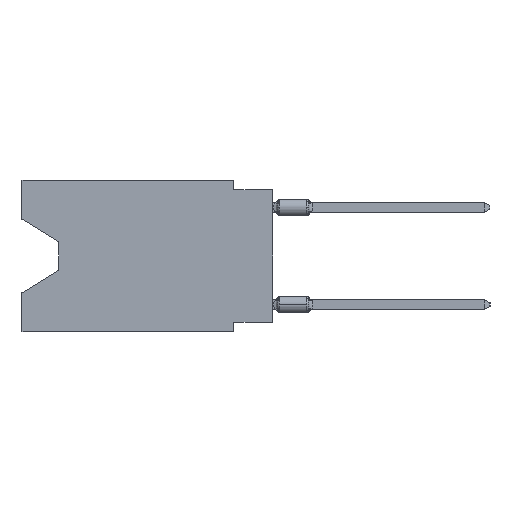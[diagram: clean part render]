
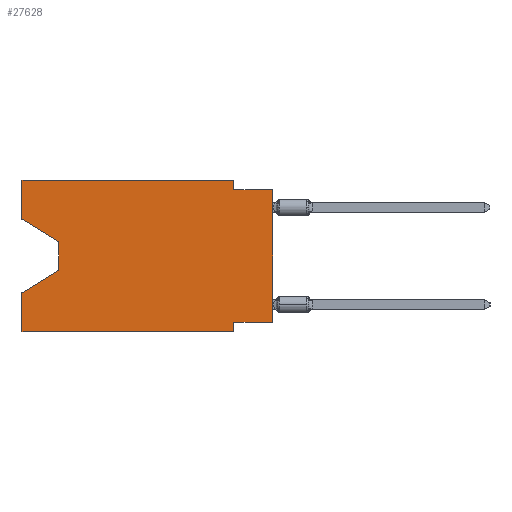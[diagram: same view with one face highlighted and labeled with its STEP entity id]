
A CAD part, left-side view. The second image highlights one B-rep face of the part: STEP entity #27628.
In plain terms, the highlighted planar face has unit normal (-1, 0, 0).
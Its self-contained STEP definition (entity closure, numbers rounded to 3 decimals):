
#30 = LINE ( 'NONE', #31520, #30660 ) ;
#579 = VECTOR ( 'NONE', #12243, 1000. ) ;
#632 = EDGE_CURVE ( 'NONE', #50674, #3811, #5623, .T. ) ;
#1959 = CARTESIAN_POINT ( 'NONE',  ( 0., 16.383, 0. ) ) ;
#2284 = VECTOR ( 'NONE', #51133, 1000. ) ;
#2565 = VERTEX_POINT ( 'NONE', #56845 ) ;
#3761 = EDGE_CURVE ( 'NONE', #54432, #61851, #59357, .T. ) ;
#3811 = VERTEX_POINT ( 'NONE', #17950 ) ;
#4368 = ORIENTED_EDGE ( 'NONE', *, *, #3761, .F. ) ;
#5499 = CARTESIAN_POINT ( 'NONE',  ( 0., 13.97, -4.013 ) ) ;
#5519 = VERTEX_POINT ( 'NONE', #28139 ) ;
#5593 = ORIENTED_EDGE ( 'NONE', *, *, #47356, .F. ) ;
#5623 = LINE ( 'NONE', #37095, #46835 ) ;
#8354 = CARTESIAN_POINT ( 'NONE',  ( 0., 0., -9.271 ) ) ;
#8778 = EDGE_CURVE ( 'NONE', #24828, #60462, #59482, .T. ) ;
#9676 = VECTOR ( 'NONE', #62360, 1000. ) ;
#9912 = CARTESIAN_POINT ( 'NONE',  ( 0., 2.54, -9.271 ) ) ;
#10044 = VECTOR ( 'NONE', #13148, 1000. ) ;
#10761 = DIRECTION ( 'NONE',  ( 0., -1., 0. ) ) ;
#10808 = EDGE_CURVE ( 'NONE', #66509, #2565, #11108, .T. ) ;
#11108 = LINE ( 'NONE', #31983, #42632 ) ;
#11508 = LINE ( 'NONE', #32378, #61722 ) ;
#11932 = ORIENTED_EDGE ( 'NONE', *, *, #10808, .F. ) ;
#12243 = DIRECTION ( 'NONE',  ( 0., 0.855, -0.519 ) ) ;
#13148 = DIRECTION ( 'NONE',  ( 0., 0., 1. ) ) ;
#14073 = AXIS2_PLACEMENT_3D ( 'NONE', #1959, #17699, #63919 ) ;
#14655 = ORIENTED_EDGE ( 'NONE', *, *, #8778, .T. ) ;
#15112 = CARTESIAN_POINT ( 'NONE',  ( 0., 16.383, 0. ) ) ;
#17358 = FACE_OUTER_BOUND ( 'NONE', #24933, .T. ) ;
#17454 = DIRECTION ( 'NONE',  ( 0., 0., -1. ) ) ;
#17462 = CARTESIAN_POINT ( 'NONE',  ( 0., 16.383, -7.36 ) ) ;
#17615 = CARTESIAN_POINT ( 'NONE',  ( 0., 16.383, 0. ) ) ;
#17699 = DIRECTION ( 'NONE',  ( 1., 0., 0. ) ) ;
#17950 = CARTESIAN_POINT ( 'NONE',  ( 0., 0., -0.635 ) ) ;
#18912 = EDGE_CURVE ( 'NONE', #53524, #24828, #31519, .T. ) ;
#21018 = EDGE_CURVE ( 'NONE', #23664, #53524, #61059, .T. ) ;
#21245 = LINE ( 'NONE', #15112, #24040 ) ;
#22014 = EDGE_CURVE ( 'NONE', #23664, #66509, #60040, .T. ) ;
#22444 = DIRECTION ( 'NONE',  ( 0., -1., 0. ) ) ;
#23127 = CARTESIAN_POINT ( 'NONE',  ( 0., 2.54, -9.906 ) ) ;
#23664 = VERTEX_POINT ( 'NONE', #26900 ) ;
#24040 = VECTOR ( 'NONE', #46917, 1000. ) ;
#24047 = ORIENTED_EDGE ( 'NONE', *, *, #66608, .F. ) ;
#24828 = VERTEX_POINT ( 'NONE', #53212 ) ;
#24933 = EDGE_LOOP ( 'NONE', ( #55730, #25676, #14655, #5593, #41913, #36327, #4368, #30558, #41823, #24047, #11932, #35846 ) ) ;
#25676 = ORIENTED_EDGE ( 'NONE', *, *, #18912, .T. ) ;
#25753 = CARTESIAN_POINT ( 'NONE',  ( 0., 16.383, 0. ) ) ;
#26900 = CARTESIAN_POINT ( 'NONE',  ( 0., 16.383, -2.546 ) ) ;
#27628 = ADVANCED_FACE ( 'NONE', ( #17358 ), #53987, .F. ) ;
#28139 = CARTESIAN_POINT ( 'NONE',  ( 0., 16.383, -9.906 ) ) ;
#30388 = CARTESIAN_POINT ( 'NONE',  ( 0., 0., -9.271 ) ) ;
#30558 = ORIENTED_EDGE ( 'NONE', *, *, #56181, .T. ) ;
#30660 = VECTOR ( 'NONE', #63664, 1000. ) ;
#31519 = LINE ( 'NONE', #5499, #45036 ) ;
#31520 = CARTESIAN_POINT ( 'NONE',  ( 0., 2.54, -9.906 ) ) ;
#31983 = CARTESIAN_POINT ( 'NONE',  ( 0., 16.383, 0. ) ) ;
#32033 = DIRECTION ( 'NONE',  ( 0., 0., 1. ) ) ;
#32378 = CARTESIAN_POINT ( 'NONE',  ( 0., 16.383, -9.906 ) ) ;
#33342 = DIRECTION ( 'NONE',  ( 0., 1., 0. ) ) ;
#35846 = ORIENTED_EDGE ( 'NONE', *, *, #22014, .F. ) ;
#36327 = ORIENTED_EDGE ( 'NONE', *, *, #47594, .F. ) ;
#37095 = CARTESIAN_POINT ( 'NONE',  ( 0., 0., -0.635 ) ) ;
#37155 = CARTESIAN_POINT ( 'NONE',  ( 0., 0., 0. ) ) ;
#41303 = CARTESIAN_POINT ( 'NONE',  ( 0., 2.54, -0.635 ) ) ;
#41823 = ORIENTED_EDGE ( 'NONE', *, *, #632, .F. ) ;
#41913 = ORIENTED_EDGE ( 'NONE', *, *, #56097, .T. ) ;
#42632 = VECTOR ( 'NONE', #52862, 1000. ) ;
#45036 = VECTOR ( 'NONE', #17454, 1000. ) ;
#45601 = CARTESIAN_POINT ( 'NONE',  ( 0., 2.54, 0. ) ) ;
#45640 = CARTESIAN_POINT ( 'NONE',  ( 0., 16.383, -2.546 ) ) ;
#46835 = VECTOR ( 'NONE', #10761, 1000. ) ;
#46917 = DIRECTION ( 'NONE',  ( 0., 0., 1. ) ) ;
#47356 = EDGE_CURVE ( 'NONE', #5519, #60462, #21245, .T. ) ;
#47594 = EDGE_CURVE ( 'NONE', #61851, #62548, #30, .T. ) ;
#50674 = VERTEX_POINT ( 'NONE', #41303 ) ;
#51133 = DIRECTION ( 'NONE',  ( 0., -0.855, -0.519 ) ) ;
#51892 = VECTOR ( 'NONE', #32033, 1000. ) ;
#52862 = DIRECTION ( 'NONE',  ( 0., -1., 0. ) ) ;
#53212 = CARTESIAN_POINT ( 'NONE',  ( 0., 13.97, -5.893 ) ) ;
#53524 = VERTEX_POINT ( 'NONE', #55627 ) ;
#53987 = PLANE ( 'NONE',  #14073 ) ;
#54432 = VERTEX_POINT ( 'NONE', #30388 ) ;
#55627 = CARTESIAN_POINT ( 'NONE',  ( 0., 13.97, -4.013 ) ) ;
#55730 = ORIENTED_EDGE ( 'NONE', *, *, #21018, .T. ) ;
#56097 = EDGE_CURVE ( 'NONE', #5519, #62548, #11508, .T. ) ;
#56181 = EDGE_CURVE ( 'NONE', #54432, #3811, #63513, .T. ) ;
#56845 = CARTESIAN_POINT ( 'NONE',  ( 0., 2.54, 0. ) ) ;
#59357 = LINE ( 'NONE', #8354, #59627 ) ;
#59482 = LINE ( 'NONE', #64268, #579 ) ;
#59627 = VECTOR ( 'NONE', #33342, 1000. ) ;
#60040 = LINE ( 'NONE', #17615, #10044 ) ;
#60462 = VERTEX_POINT ( 'NONE', #17462 ) ;
#61059 = LINE ( 'NONE', #45640, #2284 ) ;
#61722 = VECTOR ( 'NONE', #22444, 1000. ) ;
#61851 = VERTEX_POINT ( 'NONE', #9912 ) ;
#62360 = DIRECTION ( 'NONE',  ( 0., 0., -1. ) ) ;
#62548 = VERTEX_POINT ( 'NONE', #23127 ) ;
#63513 = LINE ( 'NONE', #37155, #51892 ) ;
#63664 = DIRECTION ( 'NONE',  ( 0., 0., -1. ) ) ;
#63919 = DIRECTION ( 'NONE',  ( 0., 0., -1. ) ) ;
#64268 = CARTESIAN_POINT ( 'NONE',  ( 0., 13.97, -5.893 ) ) ;
#66478 = LINE ( 'NONE', #45601, #9676 ) ;
#66509 = VERTEX_POINT ( 'NONE', #25753 ) ;
#66608 = EDGE_CURVE ( 'NONE', #2565, #50674, #66478, .T. ) ;
